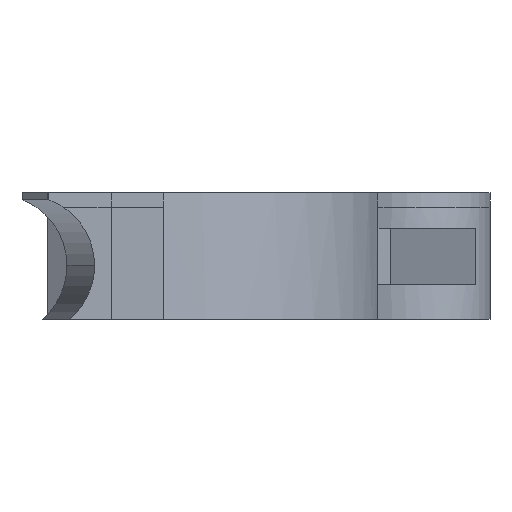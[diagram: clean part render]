
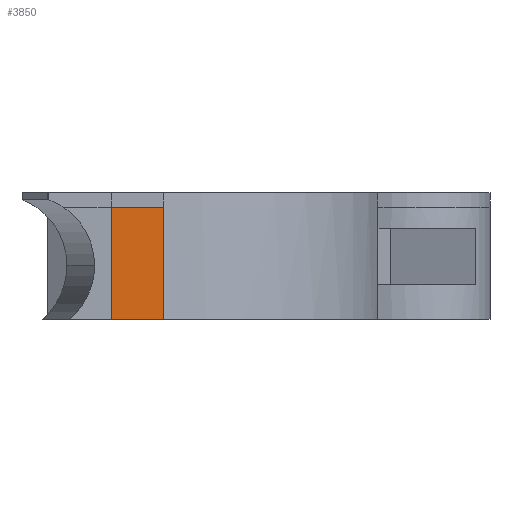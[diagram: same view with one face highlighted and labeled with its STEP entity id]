
A CAD part, left-side view. The second image highlights one B-rep face of the part: STEP entity #3850.
In plain terms, the highlighted planar face has unit normal (-1, 0, 0).
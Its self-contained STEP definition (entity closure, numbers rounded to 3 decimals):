
#691 = CYLINDRICAL_SURFACE('',#692,17.953);
#692 = AXIS2_PLACEMENT_3D('',#693,#694,#695);
#693 = CARTESIAN_POINT('',(4.789,17.741,9.05));
#694 = DIRECTION('',(0.,0.,1.));
#695 = DIRECTION('',(1.,0.,0.));
#1696 = VERTEX_POINT('',#1697);
#1697 = CARTESIAN_POINT('',(-13.,15.322,8.));
#1710 = PLANE('',#1711);
#1711 = AXIS2_PLACEMENT_3D('',#1712,#1713,#1714);
#1712 = CARTESIAN_POINT('',(-13.,23.564,8.));
#1713 = DIRECTION('',(1.,0.,0.));
#1714 = DIRECTION('',(0.,-1.,0.));
#1721 = EDGE_CURVE('',#1722,#1696,#1724,.T.);
#1722 = VERTEX_POINT('',#1723);
#1723 = CARTESIAN_POINT('',(-13.,15.322,0.));
#1724 = SURFACE_CURVE('',#1725,(#1729,#1735),.PCURVE_S1.);
#1725 = LINE('',#1726,#1727);
#1726 = CARTESIAN_POINT('',(-13.,15.322,9.05));
#1727 = VECTOR('',#1728,1.);
#1728 = DIRECTION('',(0.,0.,1.));
#1729 = PCURVE('',#691,#1730);
#1730 = DEFINITIONAL_REPRESENTATION('',(#1731),#1734);
#1731 = B_SPLINE_CURVE_WITH_KNOTS('',1,(#1732,#1733),.UNSPECIFIED.,.F.,
  .F.,(2,2),(-9.85,-0.25),.PIECEWISE_BEZIER_KNOTS.);
#1732 = CARTESIAN_POINT('',(3.277,-9.85));
#1733 = CARTESIAN_POINT('',(3.277,-0.25));
#1734 = ( GEOMETRIC_REPRESENTATION_CONTEXT(2) 
PARAMETRIC_REPRESENTATION_CONTEXT() REPRESENTATION_CONTEXT('2D SPACE',''
  ) );
#1735 = PCURVE('',#1736,#1741);
#1736 = PLANE('',#1737);
#1737 = AXIS2_PLACEMENT_3D('',#1738,#1739,#1740);
#1738 = CARTESIAN_POINT('',(-13.,0.,0.));
#1739 = DIRECTION('',(-1.,0.,0.));
#1740 = DIRECTION('',(0.,1.,0.));
#1741 = DEFINITIONAL_REPRESENTATION('',(#1742),#1745);
#1742 = B_SPLINE_CURVE_WITH_KNOTS('',1,(#1743,#1744),.UNSPECIFIED.,.F.,
  .F.,(2,2),(-9.85,-0.25),.PIECEWISE_BEZIER_KNOTS.);
#1743 = CARTESIAN_POINT('',(15.322,0.8));
#1744 = CARTESIAN_POINT('',(15.322,-8.8));
#1745 = ( GEOMETRIC_REPRESENTATION_CONTEXT(2) 
PARAMETRIC_REPRESENTATION_CONTEXT() REPRESENTATION_CONTEXT('2D SPACE',''
  ) );
#1764 = PLANE('',#1765);
#1765 = AXIS2_PLACEMENT_3D('',#1766,#1767,#1768);
#1766 = CARTESIAN_POINT('',(0.,0.,0.));
#1767 = DIRECTION('',(0.,0.,1.));
#1768 = DIRECTION('',(1.,0.,0.));
#3803 = VERTEX_POINT('',#3804);
#3804 = CARTESIAN_POINT('',(-13.,19.043,0.));
#3830 = EDGE_CURVE('',#1722,#3803,#3831,.T.);
#3831 = SURFACE_CURVE('',#3832,(#3836,#3843),.PCURVE_S1.);
#3832 = LINE('',#3833,#3834);
#3833 = CARTESIAN_POINT('',(-13.,0.,0.));
#3834 = VECTOR('',#3835,1.);
#3835 = DIRECTION('',(0.,1.,0.));
#3836 = PCURVE('',#1764,#3837);
#3837 = DEFINITIONAL_REPRESENTATION('',(#3838),#3842);
#3838 = LINE('',#3839,#3840);
#3839 = CARTESIAN_POINT('',(-13.,0.));
#3840 = VECTOR('',#3841,1.);
#3841 = DIRECTION('',(0.,1.));
#3842 = ( GEOMETRIC_REPRESENTATION_CONTEXT(2) 
PARAMETRIC_REPRESENTATION_CONTEXT() REPRESENTATION_CONTEXT('2D SPACE',''
  ) );
#3843 = PCURVE('',#1736,#3844);
#3844 = DEFINITIONAL_REPRESENTATION('',(#3845),#3849);
#3845 = LINE('',#3846,#3847);
#3846 = CARTESIAN_POINT('',(0.,0.));
#3847 = VECTOR('',#3848,1.);
#3848 = DIRECTION('',(1.,0.));
#3849 = ( GEOMETRIC_REPRESENTATION_CONTEXT(2) 
PARAMETRIC_REPRESENTATION_CONTEXT() REPRESENTATION_CONTEXT('2D SPACE',''
  ) );
#3850 = ADVANCED_FACE('',(#3851),#1736,.T.);
#3851 = FACE_BOUND('',#3852,.T.);
#3852 = EDGE_LOOP('',(#3853,#3876,#3902,#3903));
#3853 = ORIENTED_EDGE('',*,*,#3854,.F.);
#3854 = EDGE_CURVE('',#3855,#1696,#3857,.T.);
#3855 = VERTEX_POINT('',#3856);
#3856 = CARTESIAN_POINT('',(-13.,19.043,8.));
#3857 = SURFACE_CURVE('',#3858,(#3862,#3869),.PCURVE_S1.);
#3858 = LINE('',#3859,#3860);
#3859 = CARTESIAN_POINT('',(-13.,23.564,8.));
#3860 = VECTOR('',#3861,1.);
#3861 = DIRECTION('',(0.,-1.,0.));
#3862 = PCURVE('',#1736,#3863);
#3863 = DEFINITIONAL_REPRESENTATION('',(#3864),#3868);
#3864 = LINE('',#3865,#3866);
#3865 = CARTESIAN_POINT('',(23.564,-8.));
#3866 = VECTOR('',#3867,1.);
#3867 = DIRECTION('',(-1.,0.));
#3868 = ( GEOMETRIC_REPRESENTATION_CONTEXT(2) 
PARAMETRIC_REPRESENTATION_CONTEXT() REPRESENTATION_CONTEXT('2D SPACE',''
  ) );
#3869 = PCURVE('',#1710,#3870);
#3870 = DEFINITIONAL_REPRESENTATION('',(#3871),#3875);
#3871 = LINE('',#3872,#3873);
#3872 = CARTESIAN_POINT('',(0.,0.));
#3873 = VECTOR('',#3874,1.);
#3874 = DIRECTION('',(1.,0.));
#3875 = ( GEOMETRIC_REPRESENTATION_CONTEXT(2) 
PARAMETRIC_REPRESENTATION_CONTEXT() REPRESENTATION_CONTEXT('2D SPACE',''
  ) );
#3876 = ORIENTED_EDGE('',*,*,#3877,.T.);
#3877 = EDGE_CURVE('',#3855,#3803,#3878,.T.);
#3878 = SURFACE_CURVE('',#3879,(#3883,#3890),.PCURVE_S1.);
#3879 = LINE('',#3880,#3881);
#3880 = CARTESIAN_POINT('',(-13.,19.043,9.05));
#3881 = VECTOR('',#3882,1.);
#3882 = DIRECTION('',(0.,0.,-1.));
#3883 = PCURVE('',#1736,#3884);
#3884 = DEFINITIONAL_REPRESENTATION('',(#3885),#3889);
#3885 = LINE('',#3886,#3887);
#3886 = CARTESIAN_POINT('',(19.043,-9.05));
#3887 = VECTOR('',#3888,1.);
#3888 = DIRECTION('',(0.,1.));
#3889 = ( GEOMETRIC_REPRESENTATION_CONTEXT(2) 
PARAMETRIC_REPRESENTATION_CONTEXT() REPRESENTATION_CONTEXT('2D SPACE',''
  ) );
#3890 = PCURVE('',#3891,#3896);
#3891 = PLANE('',#3892);
#3892 = AXIS2_PLACEMENT_3D('',#3893,#3894,#3895);
#3893 = CARTESIAN_POINT('',(-13.,0.,0.));
#3894 = DIRECTION('',(-1.,0.,0.));
#3895 = DIRECTION('',(0.,1.,0.));
#3896 = DEFINITIONAL_REPRESENTATION('',(#3897),#3901);
#3897 = LINE('',#3898,#3899);
#3898 = CARTESIAN_POINT('',(19.043,-9.05));
#3899 = VECTOR('',#3900,1.);
#3900 = DIRECTION('',(0.,1.));
#3901 = ( GEOMETRIC_REPRESENTATION_CONTEXT(2) 
PARAMETRIC_REPRESENTATION_CONTEXT() REPRESENTATION_CONTEXT('2D SPACE',''
  ) );
#3902 = ORIENTED_EDGE('',*,*,#3830,.F.);
#3903 = ORIENTED_EDGE('',*,*,#1721,.T.);
